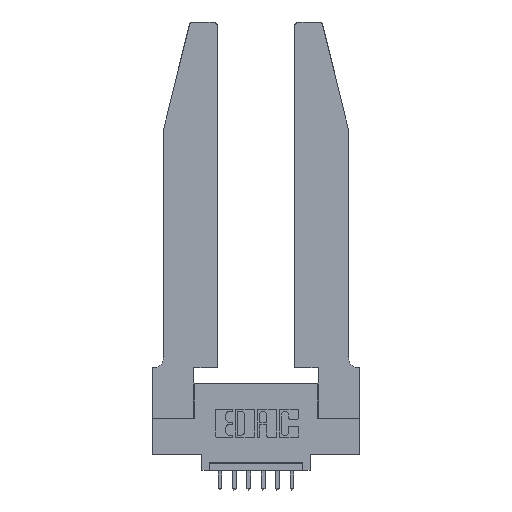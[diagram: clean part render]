
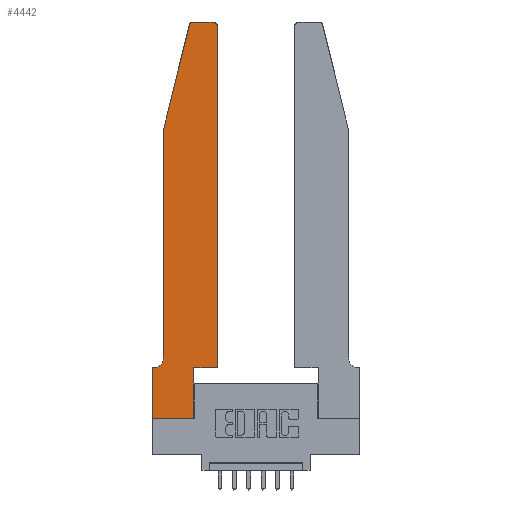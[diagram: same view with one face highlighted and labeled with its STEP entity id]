
A CAD part, top view. The second image highlights one B-rep face of the part: STEP entity #4442.
In plain terms, the highlighted planar face has unit normal (0, 0, 1).
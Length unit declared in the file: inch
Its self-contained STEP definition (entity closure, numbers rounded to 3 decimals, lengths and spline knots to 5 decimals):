
#38 = CARTESIAN_POINT ( 'NONE',  ( 0.0055, 0.35, 0.37 ) ) ;
#85 = CARTESIAN_POINT ( 'NONE',  ( 0.0755, 2., 0.37 ) ) ;
#530 = ORIENTED_EDGE ( 'NONE', *, *, #11669, .T. ) ;
#567 = VERTEX_POINT ( 'NONE', #7102 ) ;
#754 = CIRCLE ( 'NONE', #789, 0.03 ) ;
#789 = AXIS2_PLACEMENT_3D ( 'NONE', #6919, #11479, #11533 ) ;
#841 = DIRECTION ( 'NONE',  ( 1., 0., 0. ) ) ;
#1201 = ORIENTED_EDGE ( 'NONE', *, *, #1558, .T. ) ;
#1362 = ORIENTED_EDGE ( 'NONE', *, *, #2680, .T. ) ;
#1437 = DIRECTION ( 'NONE',  ( 1., 0., 0. ) ) ;
#1451 = LINE ( 'NONE', #10106, #2180 ) ;
#1558 = EDGE_CURVE ( 'NONE', #4067, #7674, #7358, .T. ) ;
#1602 = VECTOR ( 'NONE', #6588, 39.37008 ) ;
#1851 = CARTESIAN_POINT ( 'NONE',  ( 0., 0.35, 0.37 ) ) ;
#2102 = ORIENTED_EDGE ( 'NONE', *, *, #4193, .T. ) ;
#2137 = CARTESIAN_POINT ( 'NONE',  ( 0.0755, 2., 0.37 ) ) ;
#2180 = VECTOR ( 'NONE', #3441, 39.37008 ) ;
#2600 = CARTESIAN_POINT ( 'NONE',  ( 0., 0., 0.37 ) ) ;
#2611 = VECTOR ( 'NONE', #3608, 39.37008 ) ;
#2680 = EDGE_CURVE ( 'NONE', #6415, #14270, #754, .T. ) ;
#2745 = CARTESIAN_POINT ( 'NONE',  ( 0.284, 2.75, 0.37 ) ) ;
#3019 = ORIENTED_EDGE ( 'NONE', *, *, #5177, .T. ) ;
#3038 = CARTESIAN_POINT ( 'NONE',  ( 0.2865, 0.35, 0.37 ) ) ;
#3103 = EDGE_CURVE ( 'NONE', #4128, #11401, #6103, .T. ) ;
#3441 = DIRECTION ( 'NONE',  ( 0., 1., 0. ) ) ;
#3528 = DIRECTION ( 'NONE',  ( 0., 0., 1. ) ) ;
#3608 = DIRECTION ( 'NONE',  ( 0., -1., 0. ) ) ;
#3661 = VECTOR ( 'NONE', #1437, 39.37008 ) ;
#4004 = LINE ( 'NONE', #12481, #10774 ) ;
#4067 = VERTEX_POINT ( 'NONE', #38 ) ;
#4118 = CARTESIAN_POINT ( 'NONE',  ( 0., 0.35, 0.37 ) ) ;
#4128 = VERTEX_POINT ( 'NONE', #85 ) ;
#4170 = EDGE_CURVE ( 'NONE', #12892, #10881, #4004, .T. ) ;
#4193 = EDGE_CURVE ( 'NONE', #11401, #4067, #7467, .T. ) ;
#4273 = VECTOR ( 'NONE', #8441, 39.37008 ) ;
#4378 = CARTESIAN_POINT ( 'NONE',  ( 0.4505, 2.72, 0.37 ) ) ;
#4442 = ADVANCED_FACE ( 'NONE', ( #11816 ), #7379, .T. ) ;
#4687 = CARTESIAN_POINT ( 'NONE',  ( 0.284, 2.72, 0.37 ) ) ;
#4813 = VERTEX_POINT ( 'NONE', #6025 ) ;
#5158 = EDGE_CURVE ( 'NONE', #4813, #6933, #7094, .T. ) ;
#5177 = EDGE_CURVE ( 'NONE', #567, #4128, #9781, .T. ) ;
#5248 = DIRECTION ( 'NONE',  ( 0., 0., 1. ) ) ;
#5292 = VECTOR ( 'NONE', #8750, 39.37008 ) ;
#5342 = AXIS2_PLACEMENT_3D ( 'NONE', #1851, #5248, #841 ) ;
#5456 = CIRCLE ( 'NONE', #12984, 0.03 ) ;
#5547 = CARTESIAN_POINT ( 'NONE',  ( 0.4505, 0.35, 0.37 ) ) ;
#5789 = DIRECTION ( 'NONE',  ( 1., 0., 0. ) ) ;
#5797 = DIRECTION ( 'NONE',  ( -0.239, -0.971, 0. ) ) ;
#6025 = CARTESIAN_POINT ( 'NONE',  ( 0.2865, 0.35, 0.37 ) ) ;
#6103 = LINE ( 'NONE', #2137, #1602 ) ;
#6415 = VERTEX_POINT ( 'NONE', #4378 ) ;
#6588 = DIRECTION ( 'NONE',  ( 0., -1., 0. ) ) ;
#6854 = CARTESIAN_POINT ( 'NONE',  ( 0., 0., 0.37 ) ) ;
#6919 = CARTESIAN_POINT ( 'NONE',  ( 0.4205, 2.72, 0.37 ) ) ;
#6933 = VERTEX_POINT ( 'NONE', #5547 ) ;
#7094 = LINE ( 'NONE', #13463, #3661 ) ;
#7102 = CARTESIAN_POINT ( 'NONE',  ( 0.25487, 2.72718, 0.37 ) ) ;
#7358 = LINE ( 'NONE', #8394, #4273 ) ;
#7364 = EDGE_CURVE ( 'NONE', #10881, #4813, #12942, .T. ) ;
#7379 = PLANE ( 'NONE',  #5342 ) ;
#7459 = CARTESIAN_POINT ( 'NONE',  ( 0.0755, 0.42, 0.37 ) ) ;
#7467 = CIRCLE ( 'NONE', #13539, 0.07 ) ;
#7520 = CARTESIAN_POINT ( 'NONE',  ( 0.2605, 2.75, 0.37 ) ) ;
#7609 = ORIENTED_EDGE ( 'NONE', *, *, #5158, .T. ) ;
#7674 = VERTEX_POINT ( 'NONE', #4118 ) ;
#8261 = LINE ( 'NONE', #7520, #5292 ) ;
#8394 = CARTESIAN_POINT ( 'NONE',  ( 0.0755, 0.35, 0.37 ) ) ;
#8441 = DIRECTION ( 'NONE',  ( -1., 0., 0. ) ) ;
#8610 = CARTESIAN_POINT ( 'NONE',  ( 0.2865, 0., 0.37 ) ) ;
#8685 = EDGE_LOOP ( 'NONE', ( #14120, #9533, #3019, #10281, #2102, #1201, #530, #14084, #13916, #7609, #10639, #1362 ) ) ;
#8750 = DIRECTION ( 'NONE',  ( -1., 0., 0. ) ) ;
#8905 = LINE ( 'NONE', #6854, #2611 ) ;
#9196 = DIRECTION ( 'NONE',  ( 1., 0., 0. ) ) ;
#9228 = CARTESIAN_POINT ( 'NONE',  ( 0.0755, 2., 0.37 ) ) ;
#9366 = VECTOR ( 'NONE', #14057, 39.37008 ) ;
#9533 = ORIENTED_EDGE ( 'NONE', *, *, #13416, .T. ) ;
#9781 = LINE ( 'NONE', #9228, #10807 ) ;
#10106 = CARTESIAN_POINT ( 'NONE',  ( 0.4505, 0.35, 0.37 ) ) ;
#10281 = ORIENTED_EDGE ( 'NONE', *, *, #3103, .T. ) ;
#10343 = DIRECTION ( 'NONE',  ( -1., 0., 0. ) ) ;
#10639 = ORIENTED_EDGE ( 'NONE', *, *, #12556, .T. ) ;
#10774 = VECTOR ( 'NONE', #9196, 39.37008 ) ;
#10807 = VECTOR ( 'NONE', #5797, 39.37008 ) ;
#10881 = VERTEX_POINT ( 'NONE', #8610 ) ;
#11401 = VERTEX_POINT ( 'NONE', #7459 ) ;
#11479 = DIRECTION ( 'NONE',  ( 0., 0., 1. ) ) ;
#11533 = DIRECTION ( 'NONE',  ( 1., 0., 0. ) ) ;
#11669 = EDGE_CURVE ( 'NONE', #7674, #12892, #8905, .T. ) ;
#11816 = FACE_OUTER_BOUND ( 'NONE', #8685, .T. ) ;
#11897 = CARTESIAN_POINT ( 'NONE',  ( 0.4205, 2.75, 0.37 ) ) ;
#12393 = CARTESIAN_POINT ( 'NONE',  ( 0.0055, 0.42, 0.37 ) ) ;
#12481 = CARTESIAN_POINT ( 'NONE',  ( 0., 0., 0.37 ) ) ;
#12556 = EDGE_CURVE ( 'NONE', #6933, #6415, #1451, .T. ) ;
#12892 = VERTEX_POINT ( 'NONE', #2600 ) ;
#12934 = VERTEX_POINT ( 'NONE', #2745 ) ;
#12942 = LINE ( 'NONE', #3038, #9366 ) ;
#12984 = AXIS2_PLACEMENT_3D ( 'NONE', #4687, #3528, #5789 ) ;
#13149 = EDGE_CURVE ( 'NONE', #14270, #12934, #8261, .T. ) ;
#13416 = EDGE_CURVE ( 'NONE', #12934, #567, #5456, .T. ) ;
#13463 = CARTESIAN_POINT ( 'NONE',  ( 0.4505, 0.35, 0.37 ) ) ;
#13521 = DIRECTION ( 'NONE',  ( 0., 0., -1. ) ) ;
#13539 = AXIS2_PLACEMENT_3D ( 'NONE', #12393, #13521, #10343 ) ;
#13916 = ORIENTED_EDGE ( 'NONE', *, *, #7364, .T. ) ;
#14057 = DIRECTION ( 'NONE',  ( 0., 1., 0. ) ) ;
#14084 = ORIENTED_EDGE ( 'NONE', *, *, #4170, .T. ) ;
#14120 = ORIENTED_EDGE ( 'NONE', *, *, #13149, .T. ) ;
#14270 = VERTEX_POINT ( 'NONE', #11897 ) ;
